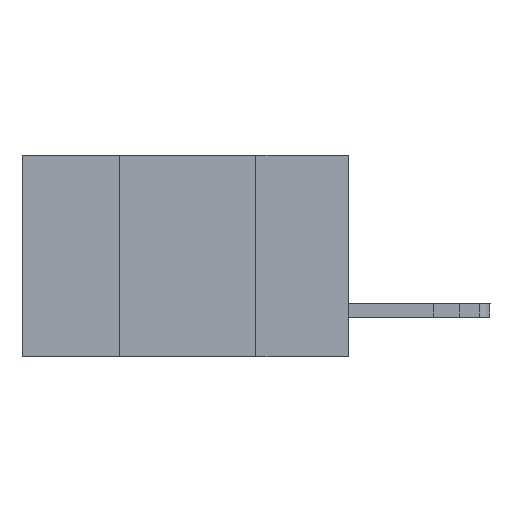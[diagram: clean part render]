
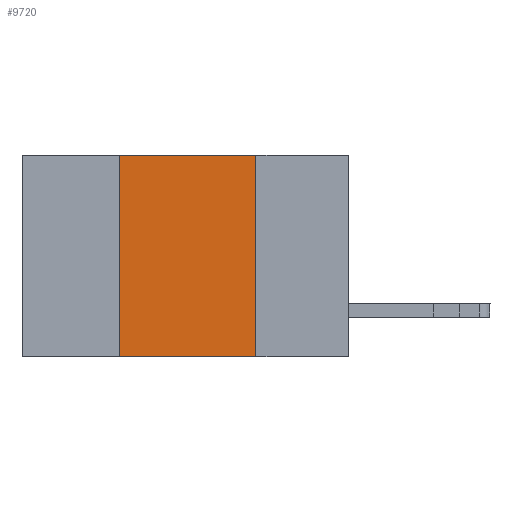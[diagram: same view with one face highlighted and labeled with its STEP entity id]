
A CAD part, left-side view. The second image highlights one B-rep face of the part: STEP entity #9720.
In plain terms, the highlighted planar face has unit normal (-1, 0, 0).
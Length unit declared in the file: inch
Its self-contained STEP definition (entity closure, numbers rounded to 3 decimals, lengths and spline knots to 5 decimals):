
#201 = AXIS2_PLACEMENT_3D ( 'NONE', #8217, #3159, #2218 ) ;
#720 = ORIENTED_EDGE ( 'NONE', *, *, #6022, .F. ) ;
#1953 = LINE ( 'NONE', #5266, #12227 ) ;
#2096 = PLANE ( 'NONE',  #201 ) ;
#2218 = DIRECTION ( 'NONE',  ( 0., 0., -1. ) ) ;
#2404 = CARTESIAN_POINT ( 'NONE',  ( 0., 0.6, 0. ) ) ;
#3159 = DIRECTION ( 'NONE',  ( 1., 0., 0. ) ) ;
#3511 = VERTEX_POINT ( 'NONE', #8703 ) ;
#3523 = ORIENTED_EDGE ( 'NONE', *, *, #4987, .T. ) ;
#3548 = VECTOR ( 'NONE', #10819, 39.37008 ) ;
#3595 = VECTOR ( 'NONE', #4447, 39.37008 ) ;
#4433 = DIRECTION ( 'NONE',  ( 0., 0., 1. ) ) ;
#4447 = DIRECTION ( 'NONE',  ( 0., 0., -1. ) ) ;
#4987 = EDGE_CURVE ( 'NONE', #9825, #12724, #10557, .T. ) ;
#5248 = DIRECTION ( 'NONE',  ( 0., -1., 0. ) ) ;
#5266 = CARTESIAN_POINT ( 'NONE',  ( 0., 0.42, 0. ) ) ;
#5406 = EDGE_LOOP ( 'NONE', ( #11134, #720, #10870, #3523 ) ) ;
#6022 = EDGE_CURVE ( 'NONE', #12615, #3511, #8999, .T. ) ;
#8217 = CARTESIAN_POINT ( 'NONE',  ( 0., 0.6, 0. ) ) ;
#8703 = CARTESIAN_POINT ( 'NONE',  ( 0., 0.17, 0. ) ) ;
#8783 = CARTESIAN_POINT ( 'NONE',  ( 0., 0.6, -0.37 ) ) ;
#8999 = LINE ( 'NONE', #2404, #9771 ) ;
#9215 = LINE ( 'NONE', #9471, #3595 ) ;
#9248 = CARTESIAN_POINT ( 'NONE',  ( 0., 0.42, 0. ) ) ;
#9471 = CARTESIAN_POINT ( 'NONE',  ( 0., 0.17, 0. ) ) ;
#9696 = CARTESIAN_POINT ( 'NONE',  ( 0., 0.17, -0.37 ) ) ;
#9720 = ADVANCED_FACE ( 'NONE', ( #9916 ), #2096, .F. ) ;
#9771 = VECTOR ( 'NONE', #5248, 39.37008 ) ;
#9825 = VERTEX_POINT ( 'NONE', #12058 ) ;
#9911 = EDGE_CURVE ( 'NONE', #9825, #12615, #1953, .T. ) ;
#9916 = FACE_OUTER_BOUND ( 'NONE', #5406, .T. ) ;
#10557 = LINE ( 'NONE', #8783, #3548 ) ;
#10819 = DIRECTION ( 'NONE',  ( 0., -1., 0. ) ) ;
#10870 = ORIENTED_EDGE ( 'NONE', *, *, #9911, .F. ) ;
#11134 = ORIENTED_EDGE ( 'NONE', *, *, #12500, .F. ) ;
#12058 = CARTESIAN_POINT ( 'NONE',  ( 0., 0.42, -0.37 ) ) ;
#12227 = VECTOR ( 'NONE', #4433, 39.37008 ) ;
#12500 = EDGE_CURVE ( 'NONE', #3511, #12724, #9215, .T. ) ;
#12615 = VERTEX_POINT ( 'NONE', #9248 ) ;
#12724 = VERTEX_POINT ( 'NONE', #9696 ) ;
